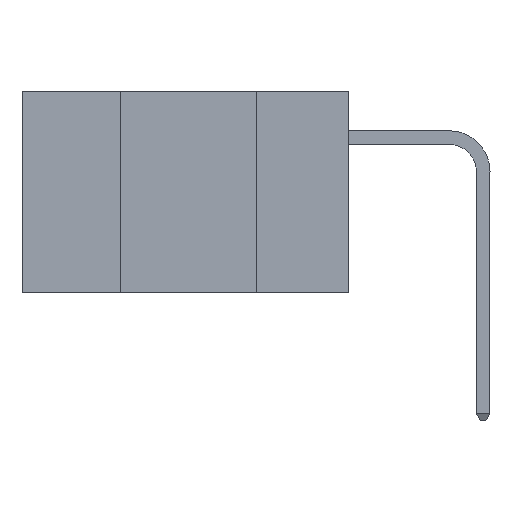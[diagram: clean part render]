
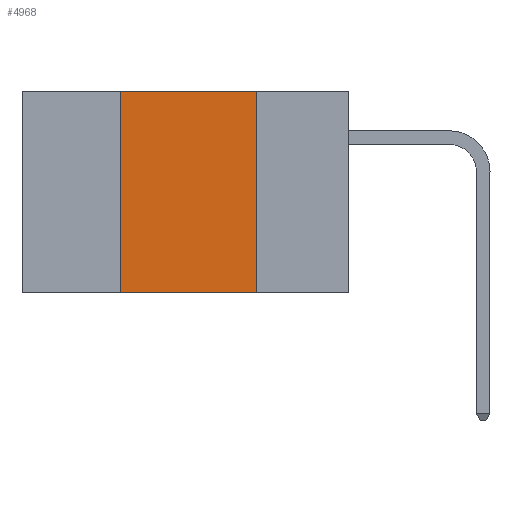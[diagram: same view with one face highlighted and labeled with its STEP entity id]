
A CAD part, left-side view. The second image highlights one B-rep face of the part: STEP entity #4968.
In plain terms, the highlighted planar face has unit normal (-1, 0, 0).
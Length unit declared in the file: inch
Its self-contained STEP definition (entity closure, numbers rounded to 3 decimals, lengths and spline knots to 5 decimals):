
#127 = CARTESIAN_POINT ( 'NONE',  ( 0., 0.6, 0. ) ) ;
#189 = PLANE ( 'NONE',  #1222 ) ;
#197 = FACE_OUTER_BOUND ( 'NONE', #7526, .T. ) ;
#489 = CARTESIAN_POINT ( 'NONE',  ( 0., 0.6, 0. ) ) ;
#1222 = AXIS2_PLACEMENT_3D ( 'NONE', #127, #1556, #1504 ) ;
#1457 = LINE ( 'NONE', #9461, #1993 ) ;
#1504 = DIRECTION ( 'NONE',  ( 0., 0., -1. ) ) ;
#1556 = DIRECTION ( 'NONE',  ( 1., 0., 0. ) ) ;
#1593 = VECTOR ( 'NONE', #9455, 39.37008 ) ;
#1993 = VECTOR ( 'NONE', #9558, 39.37008 ) ;
#2129 = CARTESIAN_POINT ( 'NONE',  ( 0., 0.42, 0. ) ) ;
#2405 = DIRECTION ( 'NONE',  ( 0., -1., 0. ) ) ;
#2947 = CARTESIAN_POINT ( 'NONE',  ( 0., 0.17, -0.37 ) ) ;
#3328 = VECTOR ( 'NONE', #7894, 39.37008 ) ;
#3445 = LINE ( 'NONE', #9436, #1593 ) ;
#3709 = LINE ( 'NONE', #4374, #3328 ) ;
#3769 = ORIENTED_EDGE ( 'NONE', *, *, #5225, .F. ) ;
#3842 = VERTEX_POINT ( 'NONE', #7438 ) ;
#4057 = VERTEX_POINT ( 'NONE', #2129 ) ;
#4251 = EDGE_CURVE ( 'NONE', #4057, #3842, #7863, .T. ) ;
#4283 = ORIENTED_EDGE ( 'NONE', *, *, #4251, .F. ) ;
#4374 = CARTESIAN_POINT ( 'NONE',  ( 0., 0.17, 0. ) ) ;
#4968 = ADVANCED_FACE ( 'NONE', ( #197 ), #189, .F. ) ;
#5052 = ORIENTED_EDGE ( 'NONE', *, *, #5272, .F. ) ;
#5174 = ORIENTED_EDGE ( 'NONE', *, *, #5292, .T. ) ;
#5225 = EDGE_CURVE ( 'NONE', #3842, #7694, #3709, .T. ) ;
#5272 = EDGE_CURVE ( 'NONE', #6638, #4057, #3445, .T. ) ;
#5292 = EDGE_CURVE ( 'NONE', #6638, #7694, #1457, .T. ) ;
#6638 = VERTEX_POINT ( 'NONE', #8712 ) ;
#7438 = CARTESIAN_POINT ( 'NONE',  ( 0., 0.17, 0. ) ) ;
#7526 = EDGE_LOOP ( 'NONE', ( #3769, #4283, #5052, #5174 ) ) ;
#7669 = VECTOR ( 'NONE', #2405, 39.37008 ) ;
#7694 = VERTEX_POINT ( 'NONE', #2947 ) ;
#7863 = LINE ( 'NONE', #489, #7669 ) ;
#7894 = DIRECTION ( 'NONE',  ( 0., 0., -1. ) ) ;
#8712 = CARTESIAN_POINT ( 'NONE',  ( 0., 0.42, -0.37 ) ) ;
#9436 = CARTESIAN_POINT ( 'NONE',  ( 0., 0.42, 0. ) ) ;
#9455 = DIRECTION ( 'NONE',  ( 0., 0., 1. ) ) ;
#9461 = CARTESIAN_POINT ( 'NONE',  ( 0., 0.6, -0.37 ) ) ;
#9558 = DIRECTION ( 'NONE',  ( 0., -1., 0. ) ) ;
